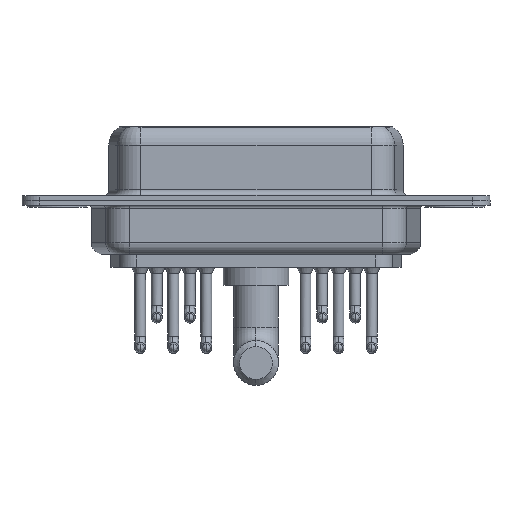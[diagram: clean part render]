
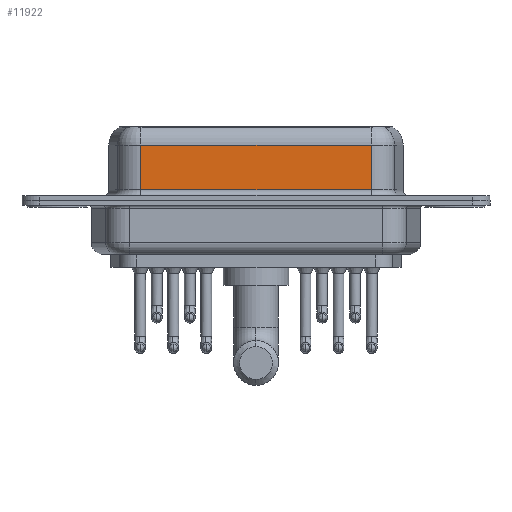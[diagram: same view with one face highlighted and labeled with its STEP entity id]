
A CAD part, front view. The second image highlights one B-rep face of the part: STEP entity #11922.
In plain terms, the highlighted planar face has unit normal (0, -1, 0).
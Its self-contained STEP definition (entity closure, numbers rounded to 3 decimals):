
#395 = DIRECTION ( 'NONE',  ( 1., 0., 0. ) ) ;
#1575 = ORIENTED_EDGE ( 'NONE', *, *, #7526, .T. ) ;
#2087 = CARTESIAN_POINT ( 'NONE',  ( 7.013, -3.95, 6.4 ) ) ;
#2900 = CARTESIAN_POINT ( 'NONE',  ( 26.287, -3.95, 0.9 ) ) ;
#4631 = VECTOR ( 'NONE', #395, 1000. ) ;
#4892 = EDGE_CURVE ( 'NONE', #15776, #15661, #14600, .T. ) ;
#5327 = LINE ( 'NONE', #16757, #8035 ) ;
#5504 = CARTESIAN_POINT ( 'NONE',  ( 26.287, -3.95, 6.4 ) ) ;
#5656 = EDGE_CURVE ( 'NONE', #11212, #7880, #11725, .T. ) ;
#5708 = CARTESIAN_POINT ( 'NONE',  ( 7.013, -3.95, 0.9 ) ) ;
#6516 = DIRECTION ( 'NONE',  ( -1., 0., 0. ) ) ;
#6529 = CARTESIAN_POINT ( 'NONE',  ( 7.013, -3.95, 4.65 ) ) ;
#6542 = VECTOR ( 'NONE', #14741, 1000. ) ;
#6684 = EDGE_LOOP ( 'NONE', ( #8906, #15376, #1575, #14440 ) ) ;
#7526 = EDGE_CURVE ( 'NONE', #7880, #15776, #9540, .T. ) ;
#7880 = VERTEX_POINT ( 'NONE', #6529 ) ;
#8035 = VECTOR ( 'NONE', #15639, 1000. ) ;
#8306 = CARTESIAN_POINT ( 'NONE',  ( 26.287, -3.95, 4.65 ) ) ;
#8336 = DIRECTION ( 'NONE',  ( 0., 0., 1. ) ) ;
#8906 = ORIENTED_EDGE ( 'NONE', *, *, #13540, .F. ) ;
#9101 = VECTOR ( 'NONE', #6516, 1000. ) ;
#9166 = CARTESIAN_POINT ( 'NONE',  ( 26.287, -3.95, 0.9 ) ) ;
#9540 = LINE ( 'NONE', #2087, #6542 ) ;
#9702 = DIRECTION ( 'NONE',  ( 0., 1., 0. ) ) ;
#10981 = FACE_OUTER_BOUND ( 'NONE', #6684, .T. ) ;
#11212 = VERTEX_POINT ( 'NONE', #8306 ) ;
#11725 = LINE ( 'NONE', #14365, #9101 ) ;
#11922 = ADVANCED_FACE ( 'NONE', ( #10981 ), #15913, .F. ) ;
#13540 = EDGE_CURVE ( 'NONE', #11212, #15661, #5327, .T. ) ;
#14004 = AXIS2_PLACEMENT_3D ( 'NONE', #5504, #9702, #8336 ) ;
#14365 = CARTESIAN_POINT ( 'NONE',  ( 26.287, -3.95, 4.65 ) ) ;
#14440 = ORIENTED_EDGE ( 'NONE', *, *, #4892, .T. ) ;
#14600 = LINE ( 'NONE', #2900, #4631 ) ;
#14741 = DIRECTION ( 'NONE',  ( 0., 0., -1. ) ) ;
#15376 = ORIENTED_EDGE ( 'NONE', *, *, #5656, .T. ) ;
#15639 = DIRECTION ( 'NONE',  ( 0., 0., -1. ) ) ;
#15661 = VERTEX_POINT ( 'NONE', #9166 ) ;
#15776 = VERTEX_POINT ( 'NONE', #5708 ) ;
#15913 = PLANE ( 'NONE',  #14004 ) ;
#16757 = CARTESIAN_POINT ( 'NONE',  ( 26.287, -3.95, 6.4 ) ) ;
